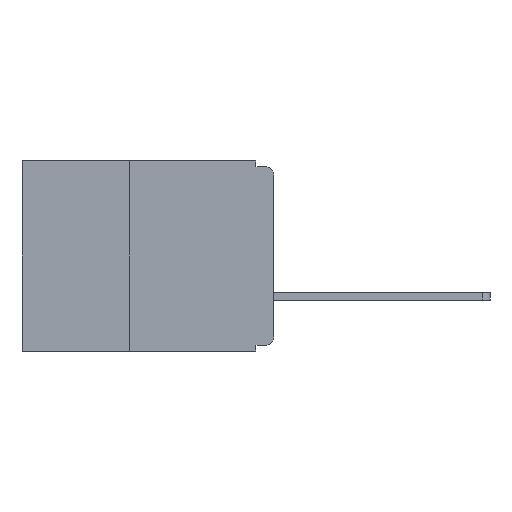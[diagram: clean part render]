
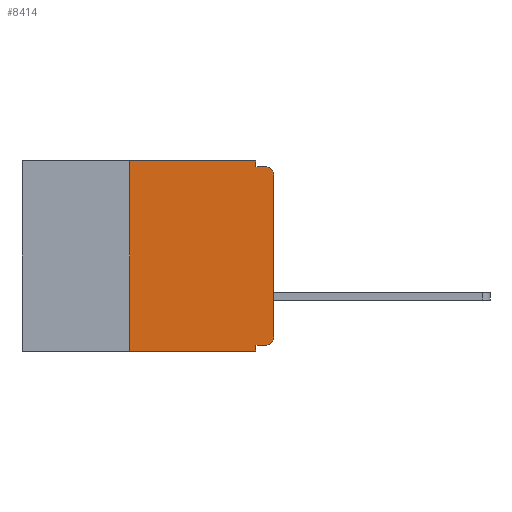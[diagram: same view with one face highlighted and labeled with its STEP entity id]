
A CAD part, left-side view. The second image highlights one B-rep face of the part: STEP entity #8414.
In plain terms, the highlighted planar face has unit normal (-1, 0, 0).
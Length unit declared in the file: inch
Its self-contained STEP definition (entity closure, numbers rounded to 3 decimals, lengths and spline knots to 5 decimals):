
#58 = VERTEX_POINT ( 'NONE', #20765 ) ;
#167 = VERTEX_POINT ( 'NONE', #17518 ) ;
#276 = ORIENTED_EDGE ( 'NONE', *, *, #1393, .T. ) ;
#504 = DIRECTION ( 'NONE',  ( 0., -1., 0. ) ) ;
#542 = ORIENTED_EDGE ( 'NONE', *, *, #21865, .T. ) ;
#875 = DIRECTION ( 'NONE',  ( 0., 0., -1. ) ) ;
#1282 = VECTOR ( 'NONE', #21983, 39.37008 ) ;
#1365 = CARTESIAN_POINT ( 'NONE',  ( 0., 0.015, -0.025 ) ) ;
#1393 = EDGE_CURVE ( 'NONE', #28231, #19270, #20483, .T. ) ;
#1684 = DIRECTION ( 'NONE',  ( 1., 0., 0. ) ) ;
#1920 = CARTESIAN_POINT ( 'NONE',  ( 0., 0.437, 0. ) ) ;
#2903 = CARTESIAN_POINT ( 'NONE',  ( 0., 0.437, 0. ) ) ;
#4194 = PLANE ( 'NONE',  #16385 ) ;
#4269 = EDGE_LOOP ( 'NONE', ( #6863, #276, #4379, #26311, #26039, #20690, #542, #13046, #19556, #24907 ) ) ;
#4379 = ORIENTED_EDGE ( 'NONE', *, *, #5575, .F. ) ;
#4512 = DIRECTION ( 'NONE',  ( 0., 0., -1. ) ) ;
#4553 = LINE ( 'NONE', #27884, #22302 ) ;
#4986 = EDGE_CURVE ( 'NONE', #6009, #28231, #18684, .T. ) ;
#5105 = CARTESIAN_POINT ( 'NONE',  ( 0., 0., -0.305 ) ) ;
#5575 = EDGE_CURVE ( 'NONE', #58, #19270, #19788, .T. ) ;
#5798 = VECTOR ( 'NONE', #8410, 39.37008 ) ;
#5986 = FACE_OUTER_BOUND ( 'NONE', #4269, .T. ) ;
#6009 = VERTEX_POINT ( 'NONE', #5105 ) ;
#6863 = ORIENTED_EDGE ( 'NONE', *, *, #4986, .T. ) ;
#8237 = CARTESIAN_POINT ( 'NONE',  ( 0., 0., 0. ) ) ;
#8410 = DIRECTION ( 'NONE',  ( 0., 0., 1. ) ) ;
#8414 = ADVANCED_FACE ( 'NONE', ( #5986 ), #4194, .F. ) ;
#10269 = DIRECTION ( 'NONE',  ( -1., 0., 0. ) ) ;
#10741 = LINE ( 'NONE', #29473, #16380 ) ;
#11739 = CARTESIAN_POINT ( 'NONE',  ( 0., 0.031, -0.33 ) ) ;
#11848 = CIRCLE ( 'NONE', #21506, 0.015 ) ;
#12563 = CARTESIAN_POINT ( 'NONE',  ( 0., 0.031, 0. ) ) ;
#12822 = EDGE_CURVE ( 'NONE', #19423, #167, #26675, .T. ) ;
#13046 = ORIENTED_EDGE ( 'NONE', *, *, #13828, .F. ) ;
#13822 = CARTESIAN_POINT ( 'NONE',  ( 0., 0., -0.025 ) ) ;
#13828 = EDGE_CURVE ( 'NONE', #17776, #30164, #21344, .T. ) ;
#13900 = VECTOR ( 'NONE', #504, 39.37008 ) ;
#14782 = CARTESIAN_POINT ( 'NONE',  ( 0., 0.015, -0.32 ) ) ;
#14966 = DIRECTION ( 'NONE',  ( 0., 0., -1. ) ) ;
#15028 = LINE ( 'NONE', #22229, #27052 ) ;
#15159 = DIRECTION ( 'NONE',  ( 0., 1., 0. ) ) ;
#16380 = VECTOR ( 'NONE', #15159, 39.37008 ) ;
#16385 = AXIS2_PLACEMENT_3D ( 'NONE', #1920, #1684, #875 ) ;
#16702 = VERTEX_POINT ( 'NONE', #24739 ) ;
#17458 = DIRECTION ( 'NONE',  ( 0., 0., -1. ) ) ;
#17518 = CARTESIAN_POINT ( 'NONE',  ( 0., 0.031, 0. ) ) ;
#17556 = EDGE_CURVE ( 'NONE', #27900, #17776, #10741, .T. ) ;
#17776 = VERTEX_POINT ( 'NONE', #20732 ) ;
#18156 = EDGE_CURVE ( 'NONE', #27900, #6009, #11848, .T. ) ;
#18684 = LINE ( 'NONE', #8237, #5798 ) ;
#19270 = VERTEX_POINT ( 'NONE', #26824 ) ;
#19423 = VERTEX_POINT ( 'NONE', #29680 ) ;
#19556 = ORIENTED_EDGE ( 'NONE', *, *, #17556, .F. ) ;
#19788 = LINE ( 'NONE', #21805, #1282 ) ;
#20483 = CIRCLE ( 'NONE', #26747, 0.015 ) ;
#20598 = VECTOR ( 'NONE', #4512, 39.37008 ) ;
#20690 = ORIENTED_EDGE ( 'NONE', *, *, #25127, .F. ) ;
#20732 = CARTESIAN_POINT ( 'NONE',  ( 0., 0.031, -0.32 ) ) ;
#20765 = CARTESIAN_POINT ( 'NONE',  ( 0., 0.031, -0.01 ) ) ;
#21344 = LINE ( 'NONE', #11739, #20598 ) ;
#21506 = AXIS2_PLACEMENT_3D ( 'NONE', #24713, #10269, #27091 ) ;
#21805 = CARTESIAN_POINT ( 'NONE',  ( 0., 0., -0.01 ) ) ;
#21865 = EDGE_CURVE ( 'NONE', #16702, #30164, #15028, .T. ) ;
#21983 = DIRECTION ( 'NONE',  ( 0., -1., 0. ) ) ;
#22229 = CARTESIAN_POINT ( 'NONE',  ( 0., 0.437, -0.33 ) ) ;
#22302 = VECTOR ( 'NONE', #25612, 39.37008 ) ;
#23271 = CARTESIAN_POINT ( 'NONE',  ( 0., 0.031, -0.33 ) ) ;
#24674 = DIRECTION ( 'NONE',  ( 0., -1., 0. ) ) ;
#24713 = CARTESIAN_POINT ( 'NONE',  ( 0., 0.015, -0.305 ) ) ;
#24739 = CARTESIAN_POINT ( 'NONE',  ( 0., 0.25, -0.33 ) ) ;
#24907 = ORIENTED_EDGE ( 'NONE', *, *, #18156, .T. ) ;
#25127 = EDGE_CURVE ( 'NONE', #16702, #19423, #4553, .T. ) ;
#25612 = DIRECTION ( 'NONE',  ( 0., 0., 1. ) ) ;
#25777 = VECTOR ( 'NONE', #14966, 39.37008 ) ;
#26039 = ORIENTED_EDGE ( 'NONE', *, *, #12822, .F. ) ;
#26311 = ORIENTED_EDGE ( 'NONE', *, *, #29843, .F. ) ;
#26534 = LINE ( 'NONE', #12563, #25777 ) ;
#26675 = LINE ( 'NONE', #2903, #13900 ) ;
#26747 = AXIS2_PLACEMENT_3D ( 'NONE', #1365, #28059, #17458 ) ;
#26824 = CARTESIAN_POINT ( 'NONE',  ( 0., 0.015, -0.01 ) ) ;
#27052 = VECTOR ( 'NONE', #24674, 39.37008 ) ;
#27091 = DIRECTION ( 'NONE',  ( 0., 0., -1. ) ) ;
#27884 = CARTESIAN_POINT ( 'NONE',  ( 0., 0.25, -0.33 ) ) ;
#27900 = VERTEX_POINT ( 'NONE', #14782 ) ;
#28059 = DIRECTION ( 'NONE',  ( -1., 0., 0. ) ) ;
#28231 = VERTEX_POINT ( 'NONE', #13822 ) ;
#29473 = CARTESIAN_POINT ( 'NONE',  ( 0., 0., -0.32 ) ) ;
#29680 = CARTESIAN_POINT ( 'NONE',  ( 0., 0.25, 0. ) ) ;
#29843 = EDGE_CURVE ( 'NONE', #167, #58, #26534, .T. ) ;
#30164 = VERTEX_POINT ( 'NONE', #23271 ) ;
